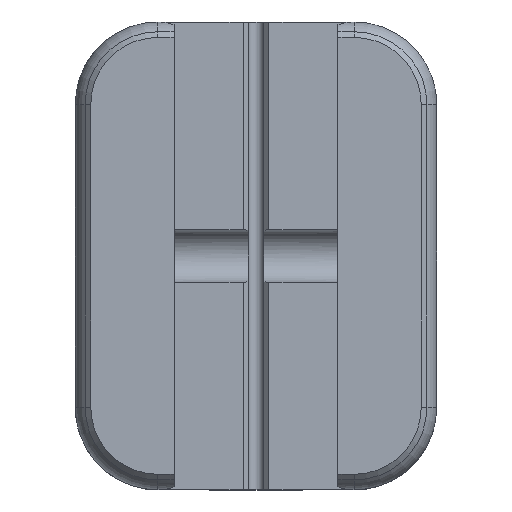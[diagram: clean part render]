
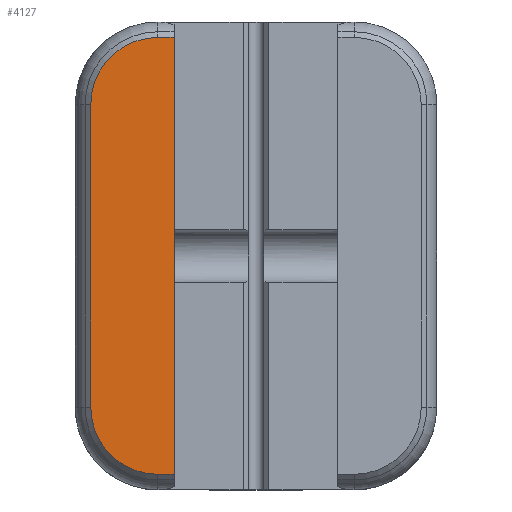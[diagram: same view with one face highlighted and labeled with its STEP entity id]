
A CAD part, top view. The second image highlights one B-rep face of the part: STEP entity #4127.
In plain terms, the highlighted planar face has unit normal (0, 0, 1).
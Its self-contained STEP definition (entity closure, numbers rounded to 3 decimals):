
#457=LINE('',#9200,#692);
#460=LINE('',#9208,#695);
#471=LINE('',#9235,#706);
#474=LINE('',#9240,#709);
#692=VECTOR('',#5491,10.);
#695=VECTOR('',#5500,10.);
#706=VECTOR('',#5529,10.);
#709=VECTOR('',#5536,10.);
#1077=FACE_OUTER_BOUND('',#1350,.T.);
#1350=EDGE_LOOP('',(#3598,#3599,#3600,#3601,#3602,#3603));
#1599=CIRCLE('',#4536,6.5);
#1600=CIRCLE('',#4539,6.5);
#1921=VERTEX_POINT('',#9192);
#1922=VERTEX_POINT('',#9194);
#1923=VERTEX_POINT('',#9198);
#1924=VERTEX_POINT('',#9202);
#1925=VERTEX_POINT('',#9206);
#1932=VERTEX_POINT('',#9234);
#2489=EDGE_CURVE('',#1921,#1922,#1599,.T.);
#2492=EDGE_CURVE('',#1923,#1921,#457,.T.);
#2494=EDGE_CURVE('',#1924,#1923,#1600,.T.);
#2496=EDGE_CURVE('',#1925,#1924,#460,.T.);
#2510=EDGE_CURVE('',#1922,#1932,#471,.T.);
#2513=EDGE_CURVE('',#1932,#1925,#474,.F.);
#3598=ORIENTED_EDGE('',*,*,#2510,.F.);
#3599=ORIENTED_EDGE('',*,*,#2489,.F.);
#3600=ORIENTED_EDGE('',*,*,#2492,.F.);
#3601=ORIENTED_EDGE('',*,*,#2494,.F.);
#3602=ORIENTED_EDGE('',*,*,#2496,.F.);
#3603=ORIENTED_EDGE('',*,*,#2513,.F.);
#3868=PLANE('',#4552);
#4127=ADVANCED_FACE('',(#1077),#3868,.F.);
#4536=AXIS2_PLACEMENT_3D('',#9195,#5485,#5486);
#4539=AXIS2_PLACEMENT_3D('',#9204,#5495,#5496);
#4552=AXIS2_PLACEMENT_3D('',#9242,#5538,#5539);
#5485=DIRECTION('center_axis',(0.,0.,
-1.));
#5486=DIRECTION('ref_axis',(-0.707,0.707,0.));
#5491=DIRECTION('',(0.,1.,0.));
#5495=DIRECTION('center_axis',(0.,0.,
-1.));
#5496=DIRECTION('ref_axis',(-0.707,-0.707,0.));
#5500=DIRECTION('',(-1.,0.,0.));
#5529=DIRECTION('',(1.,0.,0.));
#5536=DIRECTION('',(0.,1.,0.));
#5538=DIRECTION('center_axis',(0.,0.,
-1.));
#5539=DIRECTION('ref_axis',(1.,0.,0.));
#9192=CARTESIAN_POINT('',(-16.,69.653,-24.354));
#9194=CARTESIAN_POINT('',(-9.5,76.153,-24.354));
#9195=CARTESIAN_POINT('Origin',(-9.5,69.653,-24.354));
#9198=CARTESIAN_POINT('',(-16.,40.355,-24.354));
#9200=CARTESIAN_POINT('',(-16.,69.903,-24.354));
#9202=CARTESIAN_POINT('',(-9.5,33.855,-24.354));
#9204=CARTESIAN_POINT('Origin',(-9.5,40.355,-24.354));
#9206=CARTESIAN_POINT('',(-7.936,33.855,-24.354));
#9208=CARTESIAN_POINT('',(-10.135,33.855,-24.354));
#9234=CARTESIAN_POINT('',(-7.936,76.153,-24.354));
#9235=CARTESIAN_POINT('',(-10.135,76.153,-24.354));
#9240=CARTESIAN_POINT('',(-7.936,42.504,-24.354));
#9242=CARTESIAN_POINT('Origin',(-20.269,69.903,-24.354));
